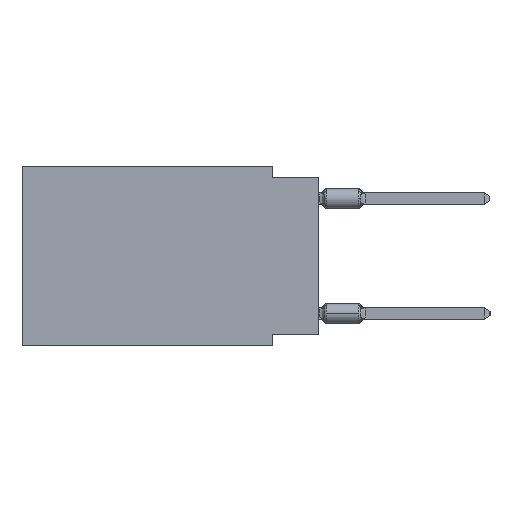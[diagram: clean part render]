
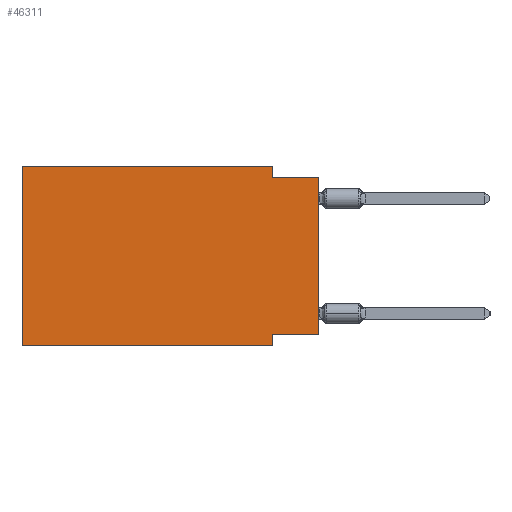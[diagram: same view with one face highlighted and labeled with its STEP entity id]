
A CAD part, left-side view. The second image highlights one B-rep face of the part: STEP entity #46311.
In plain terms, the highlighted planar face has unit normal (-1, 0, 0).
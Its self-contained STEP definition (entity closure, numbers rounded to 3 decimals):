
#761 = VERTEX_POINT ( 'NONE', #9280 ) ;
#945 = EDGE_CURVE ( 'NONE', #15848, #49710, #4203, .T. ) ;
#3649 = DIRECTION ( 'NONE',  ( 0., 0., 1. ) ) ;
#4203 = LINE ( 'NONE', #16110, #19382 ) ;
#4366 = ORIENTED_EDGE ( 'NONE', *, *, #33557, .T. ) ;
#4795 = VERTEX_POINT ( 'NONE', #33171 ) ;
#4885 = VECTOR ( 'NONE', #26456, 1000. ) ;
#5010 = EDGE_CURVE ( 'NONE', #49710, #32819, #27574, .T. ) ;
#6462 = LINE ( 'NONE', #10166, #35340 ) ;
#6983 = DIRECTION ( 'NONE',  ( 0., 0., -1. ) ) ;
#7900 = CARTESIAN_POINT ( 'NONE',  ( 0., 16.383, 0. ) ) ;
#8811 = CARTESIAN_POINT ( 'NONE',  ( 0., 16.383, 0. ) ) ;
#9280 = CARTESIAN_POINT ( 'NONE',  ( 0., 2.54, -9.906 ) ) ;
#9914 = CARTESIAN_POINT ( 'NONE',  ( 0., 0., -9.271 ) ) ;
#10166 = CARTESIAN_POINT ( 'NONE',  ( 0., 2.54, -9.906 ) ) ;
#10352 = LINE ( 'NONE', #18515, #4885 ) ;
#10476 = ORIENTED_EDGE ( 'NONE', *, *, #5010, .F. ) ;
#10974 = CARTESIAN_POINT ( 'NONE',  ( 0., 0., -9.271 ) ) ;
#11941 = VECTOR ( 'NONE', #3649, 1000. ) ;
#12298 = EDGE_CURVE ( 'NONE', #47649, #761, #6462, .T. ) ;
#12303 = DIRECTION ( 'NONE',  ( 1., 0., 0. ) ) ;
#12808 = FACE_OUTER_BOUND ( 'NONE', #19775, .T. ) ;
#14452 = CARTESIAN_POINT ( 'NONE',  ( 0., 16.383, -9.906 ) ) ;
#15728 = CARTESIAN_POINT ( 'NONE',  ( 0., 0., -0.635 ) ) ;
#15848 = VERTEX_POINT ( 'NONE', #26398 ) ;
#16110 = CARTESIAN_POINT ( 'NONE',  ( 0., 2.54, 0. ) ) ;
#16156 = ORIENTED_EDGE ( 'NONE', *, *, #16371, .F. ) ;
#16371 = EDGE_CURVE ( 'NONE', #4795, #15848, #17240, .T. ) ;
#17240 = LINE ( 'NONE', #8811, #43198 ) ;
#17885 = LINE ( 'NONE', #14452, #46525 ) ;
#18515 = CARTESIAN_POINT ( 'NONE',  ( 0., 0., 0. ) ) ;
#19382 = VECTOR ( 'NONE', #23254, 1000. ) ;
#19769 = CARTESIAN_POINT ( 'NONE',  ( 0., 16.383, -9.906 ) ) ;
#19775 = EDGE_LOOP ( 'NONE', ( #4366, #10476, #50955, #16156, #21393, #37224, #20258, #34997 ) ) ;
#20258 = ORIENTED_EDGE ( 'NONE', *, *, #12298, .F. ) ;
#21355 = VECTOR ( 'NONE', #47650, 1000. ) ;
#21393 = ORIENTED_EDGE ( 'NONE', *, *, #25641, .F. ) ;
#23254 = DIRECTION ( 'NONE',  ( 0., 0., -1. ) ) ;
#24279 = VERTEX_POINT ( 'NONE', #19769 ) ;
#25641 = EDGE_CURVE ( 'NONE', #24279, #4795, #27948, .T. ) ;
#25977 = EDGE_CURVE ( 'NONE', #24279, #761, #17885, .T. ) ;
#26398 = CARTESIAN_POINT ( 'NONE',  ( 0., 2.54, 0. ) ) ;
#26456 = DIRECTION ( 'NONE',  ( 0., 0., 1. ) ) ;
#27574 = LINE ( 'NONE', #38952, #21355 ) ;
#27948 = LINE ( 'NONE', #7900, #11941 ) ;
#31563 = VERTEX_POINT ( 'NONE', #10974 ) ;
#32617 = CARTESIAN_POINT ( 'NONE',  ( 0., 16.383, 0. ) ) ;
#32819 = VERTEX_POINT ( 'NONE', #15728 ) ;
#33171 = CARTESIAN_POINT ( 'NONE',  ( 0., 16.383, 0. ) ) ;
#33557 = EDGE_CURVE ( 'NONE', #31563, #32819, #10352, .T. ) ;
#34721 = DIRECTION ( 'NONE',  ( 0., 1., 0. ) ) ;
#34997 = ORIENTED_EDGE ( 'NONE', *, *, #37923, .F. ) ;
#35340 = VECTOR ( 'NONE', #6983, 1000. ) ;
#36268 = DIRECTION ( 'NONE',  ( 0., -1., 0. ) ) ;
#36977 = AXIS2_PLACEMENT_3D ( 'NONE', #32617, #12303, #44495 ) ;
#37224 = ORIENTED_EDGE ( 'NONE', *, *, #25977, .T. ) ;
#37923 = EDGE_CURVE ( 'NONE', #31563, #47649, #50052, .T. ) ;
#38146 = CARTESIAN_POINT ( 'NONE',  ( 0., 2.54, -9.271 ) ) ;
#38730 = DIRECTION ( 'NONE',  ( 0., -1., 0. ) ) ;
#38952 = CARTESIAN_POINT ( 'NONE',  ( 0., 0., -0.635 ) ) ;
#39164 = VECTOR ( 'NONE', #34721, 1000. ) ;
#43198 = VECTOR ( 'NONE', #36268, 1000. ) ;
#44495 = DIRECTION ( 'NONE',  ( 0., 0., -1. ) ) ;
#46311 = ADVANCED_FACE ( 'NONE', ( #12808 ), #48469, .F. ) ;
#46525 = VECTOR ( 'NONE', #38730, 1000. ) ;
#47649 = VERTEX_POINT ( 'NONE', #38146 ) ;
#47650 = DIRECTION ( 'NONE',  ( 0., -1., 0. ) ) ;
#47758 = CARTESIAN_POINT ( 'NONE',  ( 0., 2.54, -0.635 ) ) ;
#48469 = PLANE ( 'NONE',  #36977 ) ;
#49710 = VERTEX_POINT ( 'NONE', #47758 ) ;
#50052 = LINE ( 'NONE', #9914, #39164 ) ;
#50955 = ORIENTED_EDGE ( 'NONE', *, *, #945, .F. ) ;
